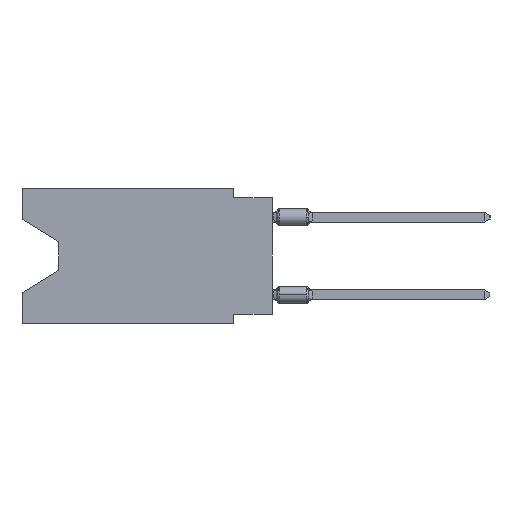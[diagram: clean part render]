
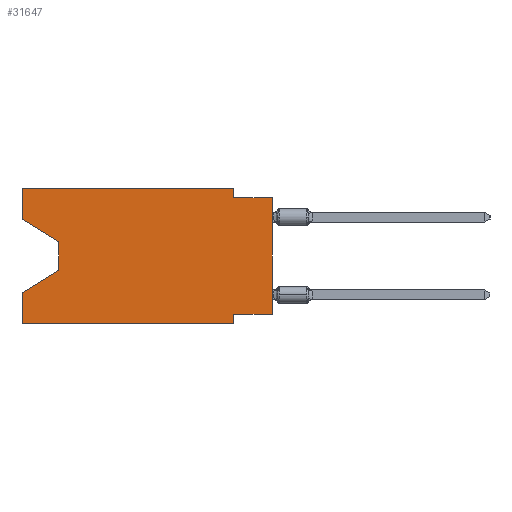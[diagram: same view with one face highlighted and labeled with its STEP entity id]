
A CAD part, left-side view. The second image highlights one B-rep face of the part: STEP entity #31647.
In plain terms, the highlighted planar face has unit normal (-1, 0, 0).
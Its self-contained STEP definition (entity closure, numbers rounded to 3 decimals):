
#127 = CARTESIAN_POINT ( 'NONE',  ( 0., 0., -0.635 ) ) ;
#141 = VECTOR ( 'NONE', #20444, 1000. ) ;
#307 = EDGE_CURVE ( 'NONE', #9002, #22733, #20092, .T. ) ;
#622 = VERTEX_POINT ( 'NONE', #40225 ) ;
#1183 = VECTOR ( 'NONE', #27451, 1000. ) ;
#1347 = EDGE_CURVE ( 'NONE', #622, #4288, #3516, .T. ) ;
#2906 = LINE ( 'NONE', #38126, #11907 ) ;
#3278 = VECTOR ( 'NONE', #23662, 1000. ) ;
#3352 = DIRECTION ( 'NONE',  ( 0., -0.855, -0.519 ) ) ;
#3400 = DIRECTION ( 'NONE',  ( 0., 0.855, -0.519 ) ) ;
#3441 = CARTESIAN_POINT ( 'NONE',  ( 0., 13.97, -3.505 ) ) ;
#3516 = LINE ( 'NONE', #10153, #41669 ) ;
#4212 = EDGE_CURVE ( 'NONE', #22733, #10831, #17584, .T. ) ;
#4288 = VERTEX_POINT ( 'NONE', #29241 ) ;
#5595 = ORIENTED_EDGE ( 'NONE', *, *, #36248, .F. ) ;
#5618 = ORIENTED_EDGE ( 'NONE', *, *, #36070, .F. ) ;
#7712 = LINE ( 'NONE', #35104, #141 ) ;
#8937 = EDGE_CURVE ( 'NONE', #34539, #28400, #2906, .T. ) ;
#9002 = VERTEX_POINT ( 'NONE', #34918 ) ;
#9792 = LINE ( 'NONE', #41823, #23445 ) ;
#9922 = VERTEX_POINT ( 'NONE', #28922 ) ;
#10045 = CARTESIAN_POINT ( 'NONE',  ( 0., 2.54, 0. ) ) ;
#10153 = CARTESIAN_POINT ( 'NONE',  ( 0., 16.383, 0. ) ) ;
#10172 = ORIENTED_EDGE ( 'NONE', *, *, #4212, .F. ) ;
#10831 = VERTEX_POINT ( 'NONE', #30889 ) ;
#10957 = DIRECTION ( 'NONE',  ( 0., 0., -1. ) ) ;
#11429 = VERTEX_POINT ( 'NONE', #36549 ) ;
#11907 = VECTOR ( 'NONE', #3352, 1000. ) ;
#12821 = DIRECTION ( 'NONE',  ( 1., 0., 0. ) ) ;
#13514 = LINE ( 'NONE', #3441, #1183 ) ;
#13710 = DIRECTION ( 'NONE',  ( 0., 1., 0. ) ) ;
#13746 = VECTOR ( 'NONE', #16906, 1000. ) ;
#13849 = ORIENTED_EDGE ( 'NONE', *, *, #15826, .T. ) ;
#13935 = LINE ( 'NONE', #27639, #17200 ) ;
#14418 = ORIENTED_EDGE ( 'NONE', *, *, #29597, .T. ) ;
#14760 = DIRECTION ( 'NONE',  ( 0., -1., 0. ) ) ;
#15826 = EDGE_CURVE ( 'NONE', #28400, #40851, #13514, .T. ) ;
#16239 = CARTESIAN_POINT ( 'NONE',  ( 0., 0., 0. ) ) ;
#16906 = DIRECTION ( 'NONE',  ( 0., 0., 1. ) ) ;
#17200 = VECTOR ( 'NONE', #3400, 1000. ) ;
#17315 = CARTESIAN_POINT ( 'NONE',  ( 0., 2.54, -8.89 ) ) ;
#17584 = LINE ( 'NONE', #42738, #25156 ) ;
#18743 = ORIENTED_EDGE ( 'NONE', *, *, #8937, .T. ) ;
#18843 = ORIENTED_EDGE ( 'NONE', *, *, #43969, .T. ) ;
#19708 = ORIENTED_EDGE ( 'NONE', *, *, #35369, .F. ) ;
#20092 = LINE ( 'NONE', #20778, #37535 ) ;
#20357 = VECTOR ( 'NONE', #13710, 1000. ) ;
#20444 = DIRECTION ( 'NONE',  ( 0., 0., 1. ) ) ;
#20778 = CARTESIAN_POINT ( 'NONE',  ( 0., 16.383, 0. ) ) ;
#20835 = ORIENTED_EDGE ( 'NONE', *, *, #1347, .F. ) ;
#22717 = VERTEX_POINT ( 'NONE', #33645 ) ;
#22733 = VERTEX_POINT ( 'NONE', #10045 ) ;
#23102 = FACE_OUTER_BOUND ( 'NONE', #43577, .T. ) ;
#23211 = LINE ( 'NONE', #37187, #3278 ) ;
#23445 = VECTOR ( 'NONE', #23738, 1000. ) ;
#23662 = DIRECTION ( 'NONE',  ( 0., -1., 0. ) ) ;
#23738 = DIRECTION ( 'NONE',  ( 0., 0., -1. ) ) ;
#24551 = DIRECTION ( 'NONE',  ( 0., 0., 1. ) ) ;
#25156 = VECTOR ( 'NONE', #10957, 1000. ) ;
#26408 = VERTEX_POINT ( 'NONE', #17315 ) ;
#26891 = ORIENTED_EDGE ( 'NONE', *, *, #33190, .F. ) ;
#27451 = DIRECTION ( 'NONE',  ( 0., 0., -1. ) ) ;
#27503 = ORIENTED_EDGE ( 'NONE', *, *, #38982, .T. ) ;
#27639 = CARTESIAN_POINT ( 'NONE',  ( 0., 13.97, -5.385 ) ) ;
#28400 = VERTEX_POINT ( 'NONE', #42158 ) ;
#28922 = CARTESIAN_POINT ( 'NONE',  ( 0., 2.54, -8.255 ) ) ;
#29241 = CARTESIAN_POINT ( 'NONE',  ( 0., 16.383, -6.852 ) ) ;
#29597 = EDGE_CURVE ( 'NONE', #622, #26408, #23211, .T. ) ;
#30418 = CARTESIAN_POINT ( 'NONE',  ( 0., 16.383, 0. ) ) ;
#30668 = CARTESIAN_POINT ( 'NONE',  ( 0., 13.97, -5.385 ) ) ;
#30872 = LINE ( 'NONE', #31091, #20357 ) ;
#30889 = CARTESIAN_POINT ( 'NONE',  ( 0., 2.54, -0.635 ) ) ;
#31091 = CARTESIAN_POINT ( 'NONE',  ( 0., 0., -8.255 ) ) ;
#31647 = ADVANCED_FACE ( 'NONE', ( #23102 ), #37074, .F. ) ;
#33190 = EDGE_CURVE ( 'NONE', #11429, #9922, #30872, .T. ) ;
#33381 = LINE ( 'NONE', #16239, #13746 ) ;
#33645 = CARTESIAN_POINT ( 'NONE',  ( 0., 0., -0.635 ) ) ;
#34077 = DIRECTION ( 'NONE',  ( 0., 0., -1. ) ) ;
#34539 = VERTEX_POINT ( 'NONE', #35668 ) ;
#34918 = CARTESIAN_POINT ( 'NONE',  ( 0., 16.383, 0. ) ) ;
#35024 = AXIS2_PLACEMENT_3D ( 'NONE', #30418, #12821, #34077 ) ;
#35104 = CARTESIAN_POINT ( 'NONE',  ( 0., 16.383, 0. ) ) ;
#35369 = EDGE_CURVE ( 'NONE', #10831, #22717, #38784, .T. ) ;
#35668 = CARTESIAN_POINT ( 'NONE',  ( 0., 16.383, -2.038 ) ) ;
#36070 = EDGE_CURVE ( 'NONE', #9922, #26408, #9792, .T. ) ;
#36248 = EDGE_CURVE ( 'NONE', #34539, #9002, #7712, .T. ) ;
#36549 = CARTESIAN_POINT ( 'NONE',  ( 0., 0., -8.255 ) ) ;
#37074 = PLANE ( 'NONE',  #35024 ) ;
#37187 = CARTESIAN_POINT ( 'NONE',  ( 0., 16.383, -8.89 ) ) ;
#37535 = VECTOR ( 'NONE', #41162, 1000. ) ;
#38126 = CARTESIAN_POINT ( 'NONE',  ( 0., 16.383, -2.038 ) ) ;
#38784 = LINE ( 'NONE', #127, #44625 ) ;
#38982 = EDGE_CURVE ( 'NONE', #11429, #22717, #33381, .T. ) ;
#40225 = CARTESIAN_POINT ( 'NONE',  ( 0., 16.383, -8.89 ) ) ;
#40769 = ORIENTED_EDGE ( 'NONE', *, *, #307, .F. ) ;
#40851 = VERTEX_POINT ( 'NONE', #30668 ) ;
#41162 = DIRECTION ( 'NONE',  ( 0., -1., 0. ) ) ;
#41669 = VECTOR ( 'NONE', #24551, 1000. ) ;
#41823 = CARTESIAN_POINT ( 'NONE',  ( 0., 2.54, -8.89 ) ) ;
#42158 = CARTESIAN_POINT ( 'NONE',  ( 0., 13.97, -3.505 ) ) ;
#42738 = CARTESIAN_POINT ( 'NONE',  ( 0., 2.54, 0. ) ) ;
#43577 = EDGE_LOOP ( 'NONE', ( #18743, #13849, #18843, #20835, #14418, #5618, #26891, #27503, #19708, #10172, #40769, #5595 ) ) ;
#43969 = EDGE_CURVE ( 'NONE', #40851, #4288, #13935, .T. ) ;
#44625 = VECTOR ( 'NONE', #14760, 1000. ) ;
